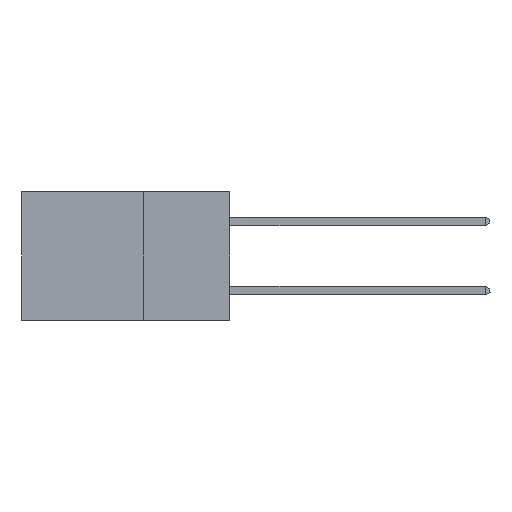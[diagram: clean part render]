
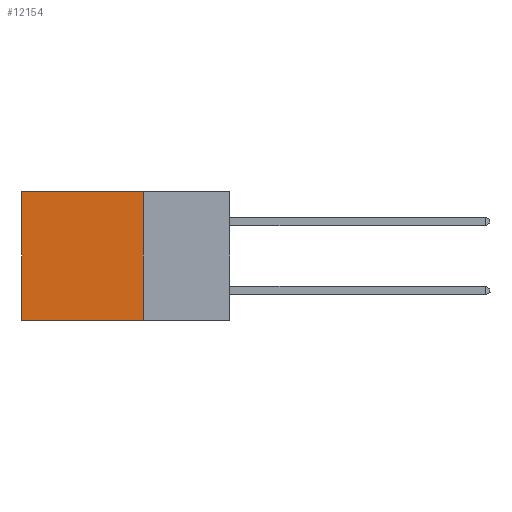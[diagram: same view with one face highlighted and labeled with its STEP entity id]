
A CAD part, left-side view. The second image highlights one B-rep face of the part: STEP entity #12154.
In plain terms, the highlighted planar face has unit normal (-1, 0, 0).
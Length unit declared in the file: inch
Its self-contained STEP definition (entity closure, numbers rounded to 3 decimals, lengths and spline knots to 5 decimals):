
#53 = ORIENTED_EDGE ( 'NONE', *, *, #13093, .T. ) ;
#490 = VERTEX_POINT ( 'NONE', #1764 ) ;
#505 = CARTESIAN_POINT ( 'NONE',  ( 0.298, 0.25, 0. ) ) ;
#513 = CARTESIAN_POINT ( 'NONE',  ( 0.298, 0.25, -0.37 ) ) ;
#852 = VERTEX_POINT ( 'NONE', #7984 ) ;
#1246 = VECTOR ( 'NONE', #1897, 39.37008 ) ;
#1764 = CARTESIAN_POINT ( 'NONE',  ( 0.298, 0.6, 0. ) ) ;
#1845 = CARTESIAN_POINT ( 'NONE',  ( 0.298, 0.6, 0. ) ) ;
#1897 = DIRECTION ( 'NONE',  ( 0., 0., -1. ) ) ;
#2392 = VECTOR ( 'NONE', #8582, 39.37008 ) ;
#2551 = AXIS2_PLACEMENT_3D ( 'NONE', #10538, #5861, #9467 ) ;
#2561 = EDGE_CURVE ( 'NONE', #13470, #8161, #2842, .T. ) ;
#2842 = LINE ( 'NONE', #10686, #8249 ) ;
#2954 = CARTESIAN_POINT ( 'NONE',  ( 0.298, 0.25, 0. ) ) ;
#3798 = CARTESIAN_POINT ( 'NONE',  ( 0.298, 0.6, -0.37 ) ) ;
#4145 = ORIENTED_EDGE ( 'NONE', *, *, #2561, .F. ) ;
#5434 = LINE ( 'NONE', #505, #2392 ) ;
#5861 = DIRECTION ( 'NONE',  ( 1., 0., 0. ) ) ;
#6020 = VECTOR ( 'NONE', #14755, 39.37008 ) ;
#7326 = FACE_OUTER_BOUND ( 'NONE', #11330, .T. ) ;
#7984 = CARTESIAN_POINT ( 'NONE',  ( 0.298, 0.25, 0. ) ) ;
#8161 = VERTEX_POINT ( 'NONE', #3798 ) ;
#8249 = VECTOR ( 'NONE', #9661, 39.37008 ) ;
#8300 = PLANE ( 'NONE',  #2551 ) ;
#8582 = DIRECTION ( 'NONE',  ( 0., 0., -1. ) ) ;
#9467 = DIRECTION ( 'NONE',  ( 0., 0., -1. ) ) ;
#9661 = DIRECTION ( 'NONE',  ( 0., 1., 0. ) ) ;
#10296 = EDGE_CURVE ( 'NONE', #490, #8161, #12444, .T. ) ;
#10538 = CARTESIAN_POINT ( 'NONE',  ( 0.298, 0.25, 0. ) ) ;
#10582 = LINE ( 'NONE', #2954, #6020 ) ;
#10686 = CARTESIAN_POINT ( 'NONE',  ( 0.298, 0.25, -0.37 ) ) ;
#11330 = EDGE_LOOP ( 'NONE', ( #13151, #4145, #13160, #53 ) ) ;
#12154 = ADVANCED_FACE ( 'NONE', ( #7326 ), #8300, .F. ) ;
#12444 = LINE ( 'NONE', #1845, #1246 ) ;
#13093 = EDGE_CURVE ( 'NONE', #852, #490, #10582, .T. ) ;
#13151 = ORIENTED_EDGE ( 'NONE', *, *, #10296, .T. ) ;
#13160 = ORIENTED_EDGE ( 'NONE', *, *, #14827, .F. ) ;
#13470 = VERTEX_POINT ( 'NONE', #513 ) ;
#14755 = DIRECTION ( 'NONE',  ( 0., 1., 0. ) ) ;
#14827 = EDGE_CURVE ( 'NONE', #852, #13470, #5434, .T. ) ;
